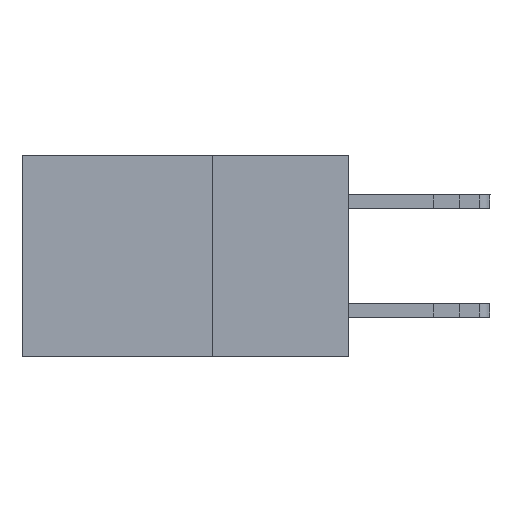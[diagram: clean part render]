
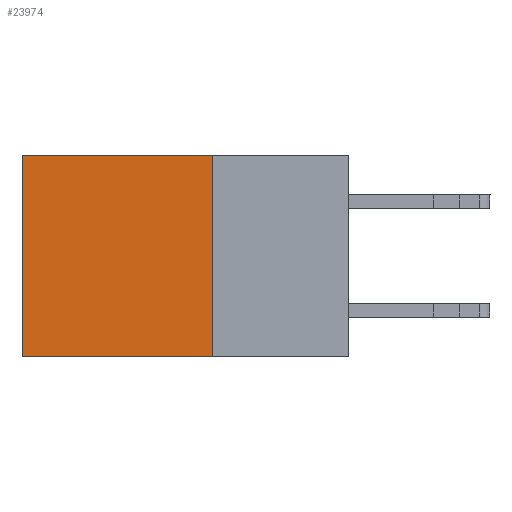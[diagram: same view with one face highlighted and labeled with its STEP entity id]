
A CAD part, left-side view. The second image highlights one B-rep face of the part: STEP entity #23974.
In plain terms, the highlighted planar face has unit normal (-1, 0, 0).
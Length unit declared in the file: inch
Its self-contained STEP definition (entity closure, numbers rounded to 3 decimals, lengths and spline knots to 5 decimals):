
#2485 = CARTESIAN_POINT ( 'NONE',  ( 0.298, 0.6, 0. ) ) ;
#2579 = DIRECTION ( 'NONE',  ( 0., 1., 0. ) ) ;
#2749 = CARTESIAN_POINT ( 'NONE',  ( 0.298, 0.25, 0. ) ) ;
#4609 = CARTESIAN_POINT ( 'NONE',  ( 0.298, 0.25, -0.37 ) ) ;
#4685 = DIRECTION ( 'NONE',  ( 0., 0., -1. ) ) ;
#5013 = LINE ( 'NONE', #4609, #9062 ) ;
#7626 = DIRECTION ( 'NONE',  ( 0., 0., -1. ) ) ;
#8084 = ORIENTED_EDGE ( 'NONE', *, *, #26220, .F. ) ;
#8439 = ORIENTED_EDGE ( 'NONE', *, *, #11523, .T. ) ;
#8569 = LINE ( 'NONE', #14801, #25596 ) ;
#8624 = VERTEX_POINT ( 'NONE', #10502 ) ;
#8998 = DIRECTION ( 'NONE',  ( 1., 0., 0. ) ) ;
#9062 = VECTOR ( 'NONE', #2579, 39.37008 ) ;
#9529 = EDGE_LOOP ( 'NONE', ( #13958, #8084, #17293, #8439 ) ) ;
#10414 = EDGE_CURVE ( 'NONE', #22630, #10548, #8569, .T. ) ;
#10502 = CARTESIAN_POINT ( 'NONE',  ( 0.298, 0.6, -0.37 ) ) ;
#10548 = VERTEX_POINT ( 'NONE', #13440 ) ;
#10763 = FACE_OUTER_BOUND ( 'NONE', #9529, .T. ) ;
#11523 = EDGE_CURVE ( 'NONE', #22630, #22429, #18160, .T. ) ;
#11878 = EDGE_CURVE ( 'NONE', #22429, #8624, #21571, .T. ) ;
#13440 = CARTESIAN_POINT ( 'NONE',  ( 0.298, 0.25, -0.37 ) ) ;
#13958 = ORIENTED_EDGE ( 'NONE', *, *, #11878, .T. ) ;
#14666 = DIRECTION ( 'NONE',  ( 0., 0., -1. ) ) ;
#14801 = CARTESIAN_POINT ( 'NONE',  ( 0.298, 0.25, 0. ) ) ;
#17293 = ORIENTED_EDGE ( 'NONE', *, *, #10414, .F. ) ;
#18160 = LINE ( 'NONE', #24796, #22144 ) ;
#19255 = PLANE ( 'NONE',  #23640 ) ;
#19542 = CARTESIAN_POINT ( 'NONE',  ( 0.298, 0.6, 0. ) ) ;
#20448 = DIRECTION ( 'NONE',  ( 0., 1., 0. ) ) ;
#21571 = LINE ( 'NONE', #19542, #23032 ) ;
#22144 = VECTOR ( 'NONE', #20448, 39.37008 ) ;
#22429 = VERTEX_POINT ( 'NONE', #2485 ) ;
#22630 = VERTEX_POINT ( 'NONE', #2749 ) ;
#23032 = VECTOR ( 'NONE', #7626, 39.37008 ) ;
#23640 = AXIS2_PLACEMENT_3D ( 'NONE', #25365, #8998, #4685 ) ;
#23974 = ADVANCED_FACE ( 'NONE', ( #10763 ), #19255, .F. ) ;
#24796 = CARTESIAN_POINT ( 'NONE',  ( 0.298, 0.25, 0. ) ) ;
#25365 = CARTESIAN_POINT ( 'NONE',  ( 0.298, 0.25, 0. ) ) ;
#25596 = VECTOR ( 'NONE', #14666, 39.37008 ) ;
#26220 = EDGE_CURVE ( 'NONE', #10548, #8624, #5013, .T. ) ;
